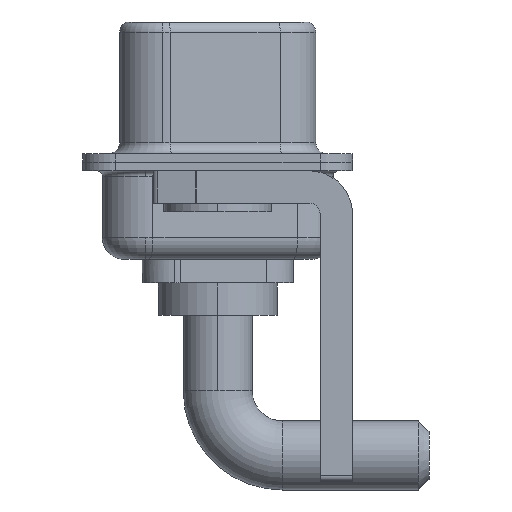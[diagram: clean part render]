
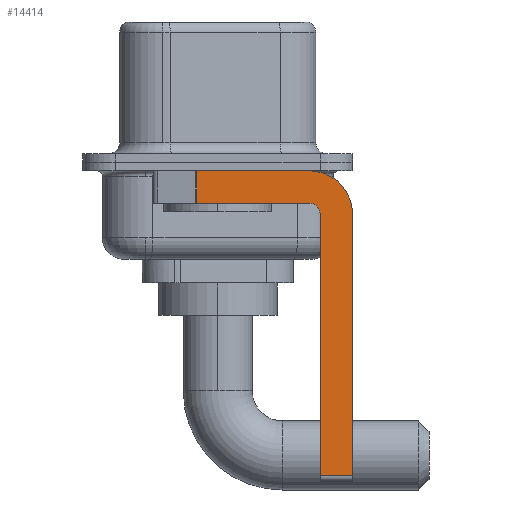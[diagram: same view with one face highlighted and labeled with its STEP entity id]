
A CAD part, left-side view. The second image highlights one B-rep face of the part: STEP entity #14414.
In plain terms, the highlighted planar face has unit normal (-1, 0, 0).
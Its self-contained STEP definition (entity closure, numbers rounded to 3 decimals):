
#130 = CARTESIAN_POINT ( 'NONE',  ( -2.9, -4.25, -1.9 ) ) ;
#275 = FACE_OUTER_BOUND ( 'NONE', #14290, .T. ) ;
#459 = VECTOR ( 'NONE', #13970, 1000. ) ;
#544 = VERTEX_POINT ( 'NONE', #15136 ) ;
#808 = VECTOR ( 'NONE', #9117, 1000. ) ;
#822 = CARTESIAN_POINT ( 'NONE',  ( -2.9, -4.75, -14.55 ) ) ;
#1009 = ORIENTED_EDGE ( 'NONE', *, *, #6969, .F. ) ;
#1210 = DIRECTION ( 'NONE',  ( 0., 0., -1. ) ) ;
#1451 = LINE ( 'NONE', #2551, #5373 ) ;
#2551 = CARTESIAN_POINT ( 'NONE',  ( -2.9, -6.25, -2.4 ) ) ;
#2951 = AXIS2_PLACEMENT_3D ( 'NONE', #4511, #14652, #10697 ) ;
#3164 = CARTESIAN_POINT ( 'NONE',  ( -2.9, -6.25, -2.4 ) ) ;
#3698 = CARTESIAN_POINT ( 'NONE',  ( -2.9, -4.25, -2.4 ) ) ;
#3946 = LINE ( 'NONE', #11380, #13573 ) ;
#4290 = CIRCLE ( 'NONE', #2951, 0.5 ) ;
#4383 = CARTESIAN_POINT ( 'NONE',  ( -2.9, -4.25, -2.4 ) ) ;
#4511 = CARTESIAN_POINT ( 'NONE',  ( -2.9, -4.25, -2.4 ) ) ;
#4864 = ORIENTED_EDGE ( 'NONE', *, *, #11470, .F. ) ;
#5049 = LINE ( 'NONE', #130, #459 ) ;
#5089 = CARTESIAN_POINT ( 'NONE',  ( -2.9, 0.978, -1.9 ) ) ;
#5107 = DIRECTION ( 'NONE',  ( 0., -1., 0. ) ) ;
#5122 = ORIENTED_EDGE ( 'NONE', *, *, #15574, .T. ) ;
#5134 = LINE ( 'NONE', #8981, #15881 ) ;
#5141 = VERTEX_POINT ( 'NONE', #822 ) ;
#5190 = CARTESIAN_POINT ( 'NONE',  ( -2.9, 0.978, -0.4 ) ) ;
#5249 = CARTESIAN_POINT ( 'NONE',  ( -2.9, -6.25, -14.55 ) ) ;
#5373 = VECTOR ( 'NONE', #1210, 1000. ) ;
#6362 = VERTEX_POINT ( 'NONE', #3164 ) ;
#6441 = CARTESIAN_POINT ( 'NONE',  ( -2.9, 3., -0.4 ) ) ;
#6969 = EDGE_CURVE ( 'NONE', #6362, #12612, #1451, .T. ) ;
#7167 = EDGE_CURVE ( 'NONE', #544, #6362, #15768, .T. ) ;
#7816 = ORIENTED_EDGE ( 'NONE', *, *, #7167, .F. ) ;
#7882 = EDGE_CURVE ( 'NONE', #11972, #14732, #8338, .T. ) ;
#8247 = AXIS2_PLACEMENT_3D ( 'NONE', #3698, #13862, #13106 ) ;
#8311 = DIRECTION ( 'NONE',  ( 0., 0., -1. ) ) ;
#8338 = LINE ( 'NONE', #14555, #11858 ) ;
#8981 = CARTESIAN_POINT ( 'NONE',  ( -2.9, -4.75, -14.8 ) ) ;
#9117 = DIRECTION ( 'NONE',  ( 0., -1., 0. ) ) ;
#9362 = DIRECTION ( 'NONE',  ( 0., 0., -1. ) ) ;
#9486 = DIRECTION ( 'NONE',  ( 1., 0., 0. ) ) ;
#9581 = CARTESIAN_POINT ( 'NONE',  ( -2.9, -4.75, -2.4 ) ) ;
#9868 = VERTEX_POINT ( 'NONE', #9992 ) ;
#9992 = CARTESIAN_POINT ( 'NONE',  ( -2.9, -4.25, -1.9 ) ) ;
#10247 = DIRECTION ( 'NONE',  ( 0., 0., 1. ) ) ;
#10459 = PLANE ( 'NONE',  #8247 ) ;
#10697 = DIRECTION ( 'NONE',  ( 0., 0., 1. ) ) ;
#11162 = ORIENTED_EDGE ( 'NONE', *, *, #7882, .T. ) ;
#11380 = CARTESIAN_POINT ( 'NONE',  ( -2.9, -4.25, -14.55 ) ) ;
#11434 = EDGE_CURVE ( 'NONE', #9868, #14732, #5049, .T. ) ;
#11470 = EDGE_CURVE ( 'NONE', #5141, #15492, #5134, .T. ) ;
#11858 = VECTOR ( 'NONE', #9362, 1000. ) ;
#11972 = VERTEX_POINT ( 'NONE', #5190 ) ;
#12612 = VERTEX_POINT ( 'NONE', #5249 ) ;
#13106 = DIRECTION ( 'NONE',  ( 0., 0., -1. ) ) ;
#13190 = ORIENTED_EDGE ( 'NONE', *, *, #11434, .F. ) ;
#13573 = VECTOR ( 'NONE', #5107, 1000. ) ;
#13862 = DIRECTION ( 'NONE',  ( 1., 0., 0. ) ) ;
#13970 = DIRECTION ( 'NONE',  ( 0., 1., 0. ) ) ;
#14171 = LINE ( 'NONE', #6441, #808 ) ;
#14260 = ORIENTED_EDGE ( 'NONE', *, *, #16213, .F. ) ;
#14290 = EDGE_LOOP ( 'NONE', ( #14260, #11162, #13190, #14672, #4864, #5122, #1009, #7816 ) ) ;
#14404 = AXIS2_PLACEMENT_3D ( 'NONE', #4383, #9486, #8311 ) ;
#14414 = ADVANCED_FACE ( 'NONE', ( #275 ), #10459, .F. ) ;
#14555 = CARTESIAN_POINT ( 'NONE',  ( -2.9, 0.978, -1.9 ) ) ;
#14652 = DIRECTION ( 'NONE',  ( -1., 0., 0. ) ) ;
#14672 = ORIENTED_EDGE ( 'NONE', *, *, #16330, .F. ) ;
#14732 = VERTEX_POINT ( 'NONE', #5089 ) ;
#15136 = CARTESIAN_POINT ( 'NONE',  ( -2.9, -4.25, -0.4 ) ) ;
#15492 = VERTEX_POINT ( 'NONE', #9581 ) ;
#15574 = EDGE_CURVE ( 'NONE', #5141, #12612, #3946, .T. ) ;
#15768 = CIRCLE ( 'NONE', #14404, 2. ) ;
#15881 = VECTOR ( 'NONE', #10247, 1000. ) ;
#16213 = EDGE_CURVE ( 'NONE', #11972, #544, #14171, .T. ) ;
#16330 = EDGE_CURVE ( 'NONE', #15492, #9868, #4290, .T. ) ;
